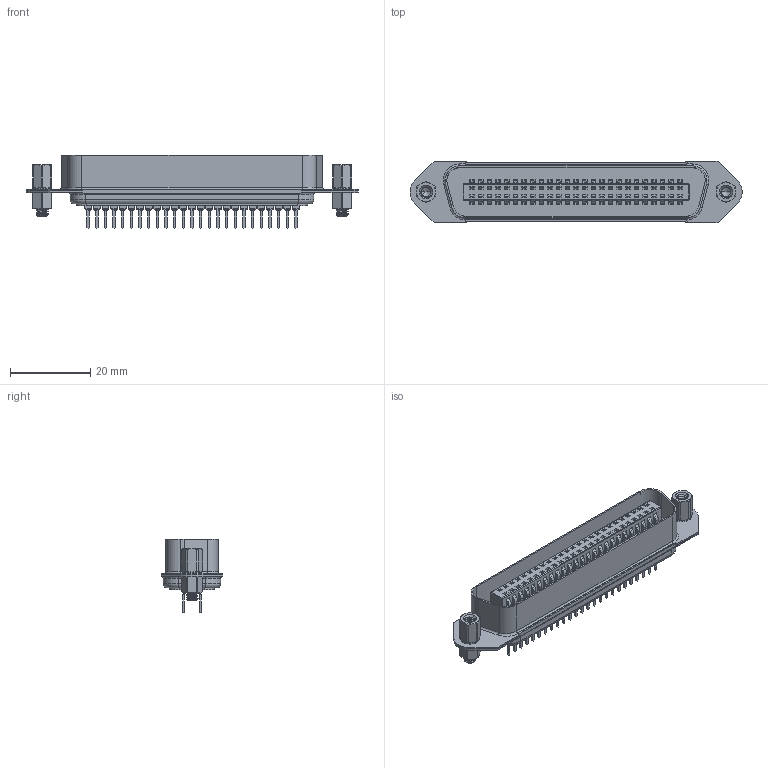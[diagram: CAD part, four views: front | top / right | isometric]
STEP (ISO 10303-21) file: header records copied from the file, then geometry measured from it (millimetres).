
FILE_DESCRIPTION (( 'STEP AP203' ), '1' );
FILE_NAME ('B57-150-621-F22.STEP', '2020-06-24T12:39:09', ( '' ), ( '' ), 'SwSTEP 2.0', 'SolidWorks 2020', '' );
FILE_SCHEMA (( 'CONFIG_CONTROL_DESIGN' ));
Length unit declared in the file: millimetre
Products named in the file (7): B57 Back Shell_50 Position; B57 Rivet_STR HEX STANDOFF; B57 Hex Standoff; B57 Front Shell MALE_50 Position UP; B57 Contacts MALE_50 Position STR; B57-150-621-F22; B57 Housing Insert MALE_50 Position UP
Assembly tree (8 placements, depth 2):
  B57-150-621-F22
    B57 Back Shell_50 Position
    B57 Rivet_STR HEX STANDOFF  x2
    B57 Housing Insert MALE_50 Position UP
    B57 Front Shell MALE_50 Position UP
    B57 Contacts MALE_50 Position STR
    B57 Hex Standoff  x2
Bounding box: 82.83 x 15.3 x 18.34 mm (x, y, z)
Volume: 6173.2 mm3; surface area: 15016.7 mm2
Topology: 57 solids, 57 shells, 5067 faces, 14329 edges, 9080 vertices
Faces by surface type: plane 3434, cylinder 1319, sphere 204, cone 62, torus 30, bspline 18
Entity records: 161686 total; most frequent: CARTESIAN_POINT 33986, ORIENTED_EDGE 27554, DIRECTION 25141, EDGE_CURVE 13777, VECTOR 10901, LINE 10901, VERTEX_POINT 8856, AXIS2_PLACEMENT_3D 7120
